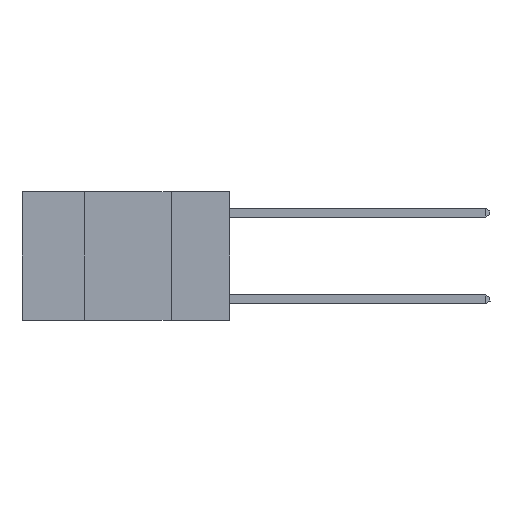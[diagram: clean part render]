
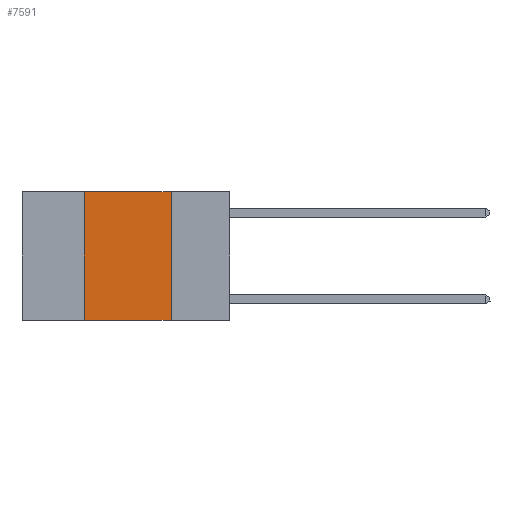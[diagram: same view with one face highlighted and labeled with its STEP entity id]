
A CAD part, left-side view. The second image highlights one B-rep face of the part: STEP entity #7591.
In plain terms, the highlighted planar face has unit normal (-1, 0, 0).
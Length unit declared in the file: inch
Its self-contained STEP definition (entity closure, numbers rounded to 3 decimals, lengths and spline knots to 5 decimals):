
#142 = CARTESIAN_POINT ( 'NONE',  ( 0., 0.17, -0.37 ) ) ;
#157 = CARTESIAN_POINT ( 'NONE',  ( 0., 0.42, 0. ) ) ;
#308 = DIRECTION ( 'NONE',  ( 0., 0., 1. ) ) ;
#859 = VERTEX_POINT ( 'NONE', #10322 ) ;
#1000 = DIRECTION ( 'NONE',  ( 1., 0., 0. ) ) ;
#1112 = LINE ( 'NONE', #8075, #2897 ) ;
#1376 = EDGE_CURVE ( 'NONE', #10313, #8146, #1112, .T. ) ;
#1514 = LINE ( 'NONE', #2904, #3817 ) ;
#1964 = EDGE_CURVE ( 'NONE', #10313, #5313, #1514, .T. ) ;
#2616 = DIRECTION ( 'NONE',  ( 0., 0., -1. ) ) ;
#2619 = FACE_OUTER_BOUND ( 'NONE', #9823, .T. ) ;
#2897 = VECTOR ( 'NONE', #308, 39.37008 ) ;
#2904 = CARTESIAN_POINT ( 'NONE',  ( 0., 0.6, -0.37 ) ) ;
#3817 = VECTOR ( 'NONE', #8839, 39.37008 ) ;
#5313 = VERTEX_POINT ( 'NONE', #142 ) ;
#5341 = VECTOR ( 'NONE', #8526, 39.37008 ) ;
#5579 = AXIS2_PLACEMENT_3D ( 'NONE', #6152, #1000, #7008 ) ;
#6152 = CARTESIAN_POINT ( 'NONE',  ( 0., 0.6, 0. ) ) ;
#6412 = ORIENTED_EDGE ( 'NONE', *, *, #9874, .F. ) ;
#6422 = EDGE_CURVE ( 'NONE', #8146, #859, #10268, .T. ) ;
#6475 = ORIENTED_EDGE ( 'NONE', *, *, #6422, .F. ) ;
#6515 = ORIENTED_EDGE ( 'NONE', *, *, #1376, .F. ) ;
#6547 = ORIENTED_EDGE ( 'NONE', *, *, #1964, .T. ) ;
#7008 = DIRECTION ( 'NONE',  ( 0., 0., -1. ) ) ;
#7223 = LINE ( 'NONE', #7735, #9420 ) ;
#7591 = ADVANCED_FACE ( 'NONE', ( #2619 ), #9476, .F. ) ;
#7686 = CARTESIAN_POINT ( 'NONE',  ( 0., 0.6, 0. ) ) ;
#7735 = CARTESIAN_POINT ( 'NONE',  ( 0., 0.17, 0. ) ) ;
#8075 = CARTESIAN_POINT ( 'NONE',  ( 0., 0.42, 0. ) ) ;
#8146 = VERTEX_POINT ( 'NONE', #157 ) ;
#8526 = DIRECTION ( 'NONE',  ( 0., -1., 0. ) ) ;
#8839 = DIRECTION ( 'NONE',  ( 0., -1., 0. ) ) ;
#9420 = VECTOR ( 'NONE', #2616, 39.37008 ) ;
#9476 = PLANE ( 'NONE',  #5579 ) ;
#9741 = CARTESIAN_POINT ( 'NONE',  ( 0., 0.42, -0.37 ) ) ;
#9823 = EDGE_LOOP ( 'NONE', ( #6412, #6475, #6515, #6547 ) ) ;
#9874 = EDGE_CURVE ( 'NONE', #859, #5313, #7223, .T. ) ;
#10268 = LINE ( 'NONE', #7686, #5341 ) ;
#10313 = VERTEX_POINT ( 'NONE', #9741 ) ;
#10322 = CARTESIAN_POINT ( 'NONE',  ( 0., 0.17, 0. ) ) ;
